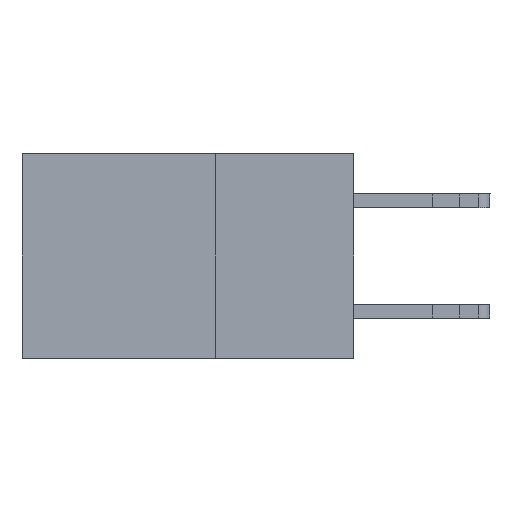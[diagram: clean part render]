
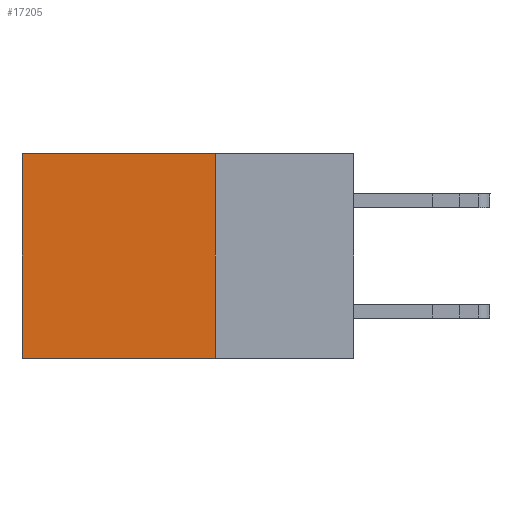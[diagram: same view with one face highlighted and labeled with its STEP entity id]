
A CAD part, left-side view. The second image highlights one B-rep face of the part: STEP entity #17205.
In plain terms, the highlighted planar face has unit normal (-1, 0, 0).
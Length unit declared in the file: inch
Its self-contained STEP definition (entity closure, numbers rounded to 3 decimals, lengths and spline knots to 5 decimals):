
#613 = CARTESIAN_POINT ( 'NONE',  ( 0.2875, 0.6, 0. ) ) ;
#1028 = ORIENTED_EDGE ( 'NONE', *, *, #13324, .T. ) ;
#1207 = CARTESIAN_POINT ( 'NONE',  ( 0.2875, 0.25, 0. ) ) ;
#1717 = DIRECTION ( 'NONE',  ( 0., 0., -1. ) ) ;
#2084 = FACE_OUTER_BOUND ( 'NONE', #10966, .T. ) ;
#2382 = VERTEX_POINT ( 'NONE', #6905 ) ;
#2540 = VERTEX_POINT ( 'NONE', #5020 ) ;
#2826 = LINE ( 'NONE', #613, #14403 ) ;
#3443 = VECTOR ( 'NONE', #1717, 39.37008 ) ;
#3574 = DIRECTION ( 'NONE',  ( 1., 0., 0. ) ) ;
#4955 = CARTESIAN_POINT ( 'NONE',  ( 0.2875, 0.25, 0. ) ) ;
#5020 = CARTESIAN_POINT ( 'NONE',  ( 0.2875, 0.25, -0.37 ) ) ;
#5092 = CARTESIAN_POINT ( 'NONE',  ( 0.2875, 0.25, 0. ) ) ;
#5118 = DIRECTION ( 'NONE',  ( 0., 0., -1. ) ) ;
#6905 = CARTESIAN_POINT ( 'NONE',  ( 0.2875, 0.6, -0.37 ) ) ;
#7225 = ORIENTED_EDGE ( 'NONE', *, *, #17180, .T. ) ;
#9095 = LINE ( 'NONE', #4955, #3443 ) ;
#9714 = CARTESIAN_POINT ( 'NONE',  ( 0.2875, 0.6, 0. ) ) ;
#10745 = EDGE_CURVE ( 'NONE', #21334, #2540, #9095, .T. ) ;
#10966 = EDGE_LOOP ( 'NONE', ( #1028, #17820, #21506, #7225 ) ) ;
#11095 = AXIS2_PLACEMENT_3D ( 'NONE', #21474, #3574, #5118 ) ;
#11277 = LINE ( 'NONE', #5092, #22372 ) ;
#11484 = DIRECTION ( 'NONE',  ( 0., 1., 0. ) ) ;
#11885 = EDGE_CURVE ( 'NONE', #2540, #2382, #18537, .T. ) ;
#12660 = DIRECTION ( 'NONE',  ( 0., 0., -1. ) ) ;
#12986 = CARTESIAN_POINT ( 'NONE',  ( 0.2875, 0.25, -0.37 ) ) ;
#13324 = EDGE_CURVE ( 'NONE', #14634, #2382, #2826, .T. ) ;
#14403 = VECTOR ( 'NONE', #12660, 39.37008 ) ;
#14634 = VERTEX_POINT ( 'NONE', #9714 ) ;
#17180 = EDGE_CURVE ( 'NONE', #21334, #14634, #11277, .T. ) ;
#17205 = ADVANCED_FACE ( 'NONE', ( #2084 ), #17531, .F. ) ;
#17531 = PLANE ( 'NONE',  #11095 ) ;
#17820 = ORIENTED_EDGE ( 'NONE', *, *, #11885, .F. ) ;
#18537 = LINE ( 'NONE', #12986, #19345 ) ;
#19345 = VECTOR ( 'NONE', #11484, 39.37008 ) ;
#21334 = VERTEX_POINT ( 'NONE', #1207 ) ;
#21474 = CARTESIAN_POINT ( 'NONE',  ( 0.2875, 0.25, 0. ) ) ;
#21506 = ORIENTED_EDGE ( 'NONE', *, *, #10745, .F. ) ;
#22267 = DIRECTION ( 'NONE',  ( 0., 1., 0. ) ) ;
#22372 = VECTOR ( 'NONE', #22267, 39.37008 ) ;
